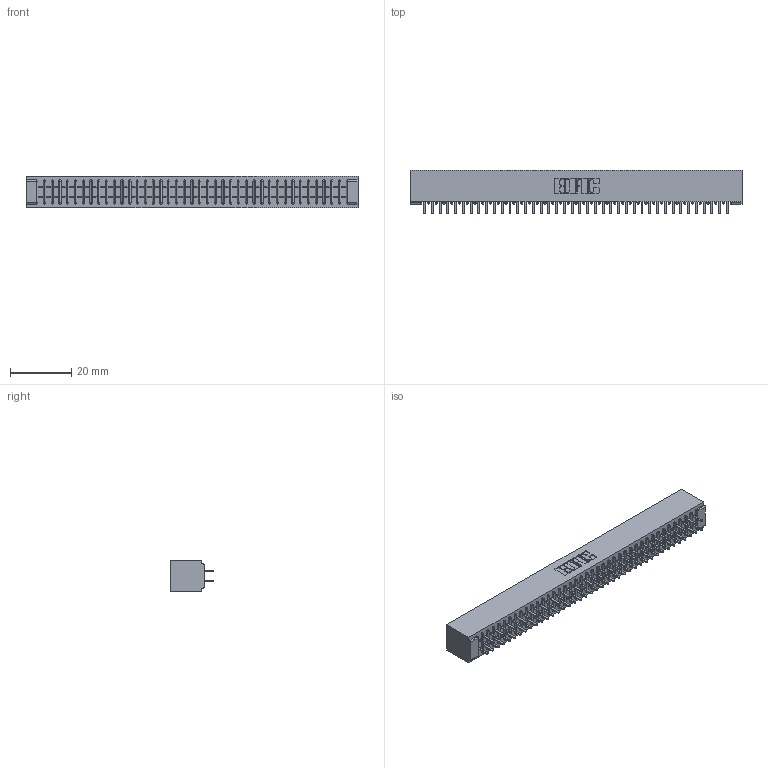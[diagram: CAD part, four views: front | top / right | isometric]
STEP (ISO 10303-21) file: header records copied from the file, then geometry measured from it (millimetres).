
FILE_DESCRIPTION (( 'STEP AP203' ), '1' );
FILE_NAME ('391-080-520-201.STEP', '2018-08-09T15:31:31', ( '' ), ( '' ), 'SwSTEP 2.0', 'SolidWorks 2016', '' );
FILE_SCHEMA (( 'CONFIG_CONTROL_DESIGN' ));
Length unit declared in the file: inch
Products named in the file (3): 341 Part_No Mounting Lugs; 341-292-001_341-292-120; 391-080-520-201
Assembly tree (81 placements, depth 2):
  391-080-520-201
    341 Part_No Mounting Lugs
    341-292-001_341-292-120  x80
Bounding box: 108.58 x 14.27 x 10.16 mm (x, y, z)
Volume: 8255.7 mm3; surface area: 15178.8 mm2
Topology: 81 solids, 81 shells, 5388 faces, 15612 edges, 10110 vertices
Faces by surface type: plane 3264, cylinder 1964, sphere 82, torus 78
Entity records: 48397 total; most frequent: CARTESIAN_POINT 8044, ORIENTED_EDGE 7992, DIRECTION 7806, EDGE_CURVE 3996, VECTOR 3230, LINE 3230, VERTEX_POINT 2526, AXIS2_PLACEMENT_3D 2288
